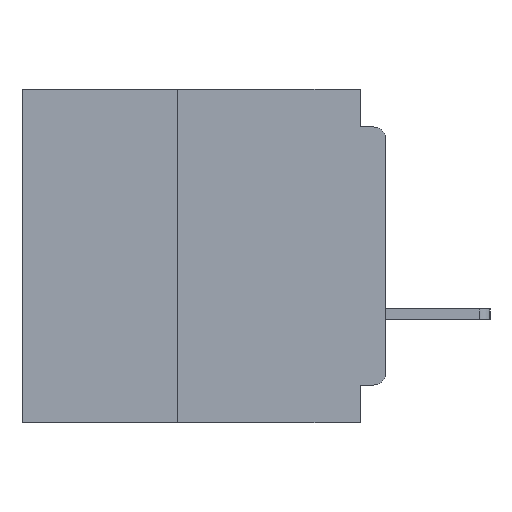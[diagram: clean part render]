
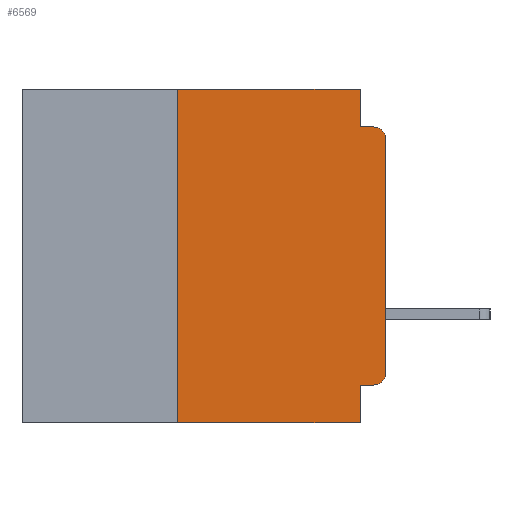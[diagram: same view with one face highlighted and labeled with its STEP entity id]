
A CAD part, left-side view. The second image highlights one B-rep face of the part: STEP entity #6569.
In plain terms, the highlighted planar face has unit normal (-1, 0, 0).
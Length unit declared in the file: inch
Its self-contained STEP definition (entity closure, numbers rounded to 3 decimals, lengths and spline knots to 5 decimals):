
#685 = EDGE_CURVE ( 'NONE', #20249, #25971, #18107, .T. ) ;
#1096 = ORIENTED_EDGE ( 'NONE', *, *, #39093, .F. ) ;
#1148 = ORIENTED_EDGE ( 'NONE', *, *, #685, .T. ) ;
#1933 = VERTEX_POINT ( 'NONE', #3880 ) ;
#2684 = CARTESIAN_POINT ( 'NONE',  ( 0., 0.015, -0.06 ) ) ;
#2809 = EDGE_CURVE ( 'NONE', #38414, #29576, #39200, .T. ) ;
#2884 = ORIENTED_EDGE ( 'NONE', *, *, #2809, .F. ) ;
#3880 = CARTESIAN_POINT ( 'NONE',  ( 0., 0.015, -0.355 ) ) ;
#4083 = FACE_OUTER_BOUND ( 'NONE', #18264, .T. ) ;
#5069 = LINE ( 'NONE', #39624, #22737 ) ;
#6184 = DIRECTION ( 'NONE',  ( 0., 0., -1. ) ) ;
#6569 = ADVANCED_FACE ( 'NONE', ( #4083 ), #31585, .F. ) ;
#7110 = ORIENTED_EDGE ( 'NONE', *, *, #15794, .F. ) ;
#9188 = DIRECTION ( 'NONE',  ( 0., -1., 0. ) ) ;
#9934 = CIRCLE ( 'NONE', #26103, 0.015 ) ;
#9952 = CARTESIAN_POINT ( 'NONE',  ( 0., 0.25, 0. ) ) ;
#10499 = DIRECTION ( 'NONE',  ( 0., 0., -1. ) ) ;
#10515 = VERTEX_POINT ( 'NONE', #26659 ) ;
#11429 = CARTESIAN_POINT ( 'NONE',  ( 0., 0., 0. ) ) ;
#11781 = ORIENTED_EDGE ( 'NONE', *, *, #27488, .T. ) ;
#11957 = EDGE_CURVE ( 'NONE', #25971, #26747, #40243, .T. ) ;
#12114 = ORIENTED_EDGE ( 'NONE', *, *, #11957, .T. ) ;
#13167 = DIRECTION ( 'NONE',  ( 0., -1., 0. ) ) ;
#13651 = CARTESIAN_POINT ( 'NONE',  ( 0., 0.437, 0. ) ) ;
#13871 = VECTOR ( 'NONE', #10499, 39.37008 ) ;
#14002 = CARTESIAN_POINT ( 'NONE',  ( 0., 0., -0.06 ) ) ;
#14661 = AXIS2_PLACEMENT_3D ( 'NONE', #2684, #27317, #6184 ) ;
#14734 = ORIENTED_EDGE ( 'NONE', *, *, #26042, .F. ) ;
#14934 = CARTESIAN_POINT ( 'NONE',  ( 0., 0.031, -0.045 ) ) ;
#15794 = EDGE_CURVE ( 'NONE', #35734, #26747, #18557, .T. ) ;
#16451 = CARTESIAN_POINT ( 'NONE',  ( 0., 0.031, -0.4 ) ) ;
#17285 = DIRECTION ( 'NONE',  ( -1., 0., 0. ) ) ;
#17456 = VECTOR ( 'NONE', #9188, 39.37008 ) ;
#18107 = LINE ( 'NONE', #11429, #34550 ) ;
#18264 = EDGE_LOOP ( 'NONE', ( #1148, #12114, #7110, #1096, #2884, #37492, #11781, #23474, #14734, #35029 ) ) ;
#18557 = LINE ( 'NONE', #33632, #17456 ) ;
#19783 = VERTEX_POINT ( 'NONE', #42129 ) ;
#19965 = DIRECTION ( 'NONE',  ( 0., 0., -1. ) ) ;
#20249 = VERTEX_POINT ( 'NONE', #41941 ) ;
#20343 = LINE ( 'NONE', #20497, #37836 ) ;
#20497 = CARTESIAN_POINT ( 'NONE',  ( 0., 0.25, -0.4 ) ) ;
#20617 = LINE ( 'NONE', #38711, #37023 ) ;
#20973 = LINE ( 'NONE', #45173, #13871 ) ;
#22737 = VECTOR ( 'NONE', #43054, 39.37008 ) ;
#22757 = EDGE_CURVE ( 'NONE', #19783, #10515, #41058, .T. ) ;
#23474 = ORIENTED_EDGE ( 'NONE', *, *, #22757, .F. ) ;
#24865 = DIRECTION ( 'NONE',  ( 0., 1., 0. ) ) ;
#25971 = VERTEX_POINT ( 'NONE', #14002 ) ;
#26042 = EDGE_CURVE ( 'NONE', #1933, #19783, #20617, .T. ) ;
#26103 = AXIS2_PLACEMENT_3D ( 'NONE', #38196, #17285, #41596 ) ;
#26659 = CARTESIAN_POINT ( 'NONE',  ( 0., 0.031, -0.4 ) ) ;
#26747 = VERTEX_POINT ( 'NONE', #28811 ) ;
#27317 = DIRECTION ( 'NONE',  ( -1., 0., 0. ) ) ;
#27488 = EDGE_CURVE ( 'NONE', #43417, #10515, #5069, .T. ) ;
#27844 = VECTOR ( 'NONE', #13167, 39.37008 ) ;
#28624 = DIRECTION ( 'NONE',  ( 0., 0., 1. ) ) ;
#28811 = CARTESIAN_POINT ( 'NONE',  ( 0., 0.015, -0.045 ) ) ;
#29576 = VERTEX_POINT ( 'NONE', #40350 ) ;
#30822 = VECTOR ( 'NONE', #19965, 39.37008 ) ;
#31296 = DIRECTION ( 'NONE',  ( 0., 0., -1. ) ) ;
#31585 = PLANE ( 'NONE',  #37598 ) ;
#31633 = CARTESIAN_POINT ( 'NONE',  ( 0., 0.437, 0. ) ) ;
#32287 = DIRECTION ( 'NONE',  ( 1., 0., 0. ) ) ;
#33632 = CARTESIAN_POINT ( 'NONE',  ( 0., 0., -0.045 ) ) ;
#34534 = EDGE_CURVE ( 'NONE', #43417, #38414, #20343, .T. ) ;
#34550 = VECTOR ( 'NONE', #28624, 39.37008 ) ;
#35029 = ORIENTED_EDGE ( 'NONE', *, *, #43135, .T. ) ;
#35734 = VERTEX_POINT ( 'NONE', #14934 ) ;
#37023 = VECTOR ( 'NONE', #24865, 39.37008 ) ;
#37492 = ORIENTED_EDGE ( 'NONE', *, *, #34534, .F. ) ;
#37598 = AXIS2_PLACEMENT_3D ( 'NONE', #31633, #32287, #31296 ) ;
#37836 = VECTOR ( 'NONE', #41311, 39.37008 ) ;
#38196 = CARTESIAN_POINT ( 'NONE',  ( 0., 0.015, -0.34 ) ) ;
#38414 = VERTEX_POINT ( 'NONE', #9952 ) ;
#38711 = CARTESIAN_POINT ( 'NONE',  ( 0., 0., -0.355 ) ) ;
#39093 = EDGE_CURVE ( 'NONE', #29576, #35734, #20973, .T. ) ;
#39200 = LINE ( 'NONE', #13651, #27844 ) ;
#39624 = CARTESIAN_POINT ( 'NONE',  ( 0., 0.437, -0.4 ) ) ;
#40243 = CIRCLE ( 'NONE', #14661, 0.015 ) ;
#40350 = CARTESIAN_POINT ( 'NONE',  ( 0., 0.031, 0. ) ) ;
#41058 = LINE ( 'NONE', #16451, #30822 ) ;
#41311 = DIRECTION ( 'NONE',  ( 0., 0., 1. ) ) ;
#41596 = DIRECTION ( 'NONE',  ( 0., 0., -1. ) ) ;
#41941 = CARTESIAN_POINT ( 'NONE',  ( 0., 0., -0.34 ) ) ;
#42129 = CARTESIAN_POINT ( 'NONE',  ( 0., 0.031, -0.355 ) ) ;
#43054 = DIRECTION ( 'NONE',  ( 0., -1., 0. ) ) ;
#43135 = EDGE_CURVE ( 'NONE', #1933, #20249, #9934, .T. ) ;
#43417 = VERTEX_POINT ( 'NONE', #43673 ) ;
#43673 = CARTESIAN_POINT ( 'NONE',  ( 0., 0.25, -0.4 ) ) ;
#45173 = CARTESIAN_POINT ( 'NONE',  ( 0., 0.031, 0. ) ) ;
